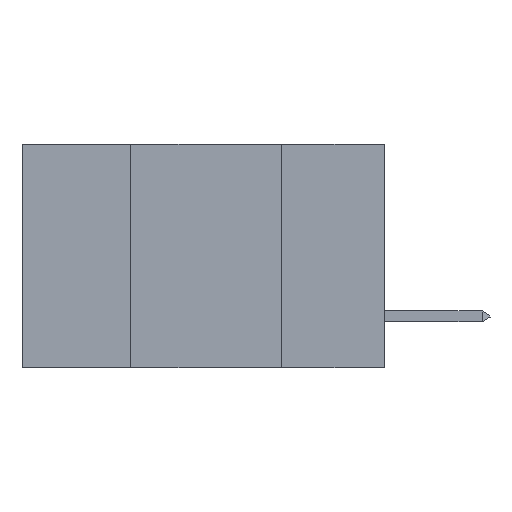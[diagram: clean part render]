
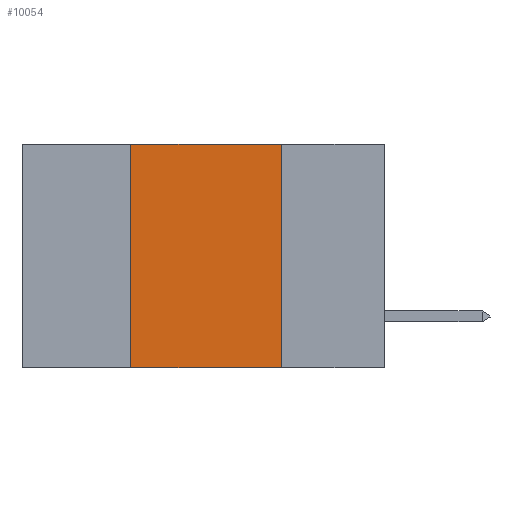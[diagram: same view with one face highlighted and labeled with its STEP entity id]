
A CAD part, left-side view. The second image highlights one B-rep face of the part: STEP entity #10054.
In plain terms, the highlighted planar face has unit normal (-1, 0, 0).
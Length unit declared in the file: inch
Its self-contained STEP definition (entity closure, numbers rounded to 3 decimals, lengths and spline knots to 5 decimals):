
#378 = DIRECTION ( 'NONE',  ( 0., -1., 0. ) ) ;
#806 = CARTESIAN_POINT ( 'NONE',  ( 0., 0.42, 0. ) ) ;
#2323 = VERTEX_POINT ( 'NONE', #33278 ) ;
#4461 = LINE ( 'NONE', #30624, #15511 ) ;
#5140 = ORIENTED_EDGE ( 'NONE', *, *, #17303, .F. ) ;
#5149 = FACE_OUTER_BOUND ( 'NONE', #28127, .T. ) ;
#9442 = VERTEX_POINT ( 'NONE', #27730 ) ;
#10054 = ADVANCED_FACE ( 'NONE', ( #5149 ), #39531, .F. ) ;
#13323 = VECTOR ( 'NONE', #378, 39.37008 ) ;
#13981 = DIRECTION ( 'NONE',  ( 0., 0., -1. ) ) ;
#13982 = CARTESIAN_POINT ( 'NONE',  ( 0., 0.6, 0. ) ) ;
#14149 = VERTEX_POINT ( 'NONE', #40591 ) ;
#14695 = DIRECTION ( 'NONE',  ( 0., 0., -1. ) ) ;
#15511 = VECTOR ( 'NONE', #14695, 39.37008 ) ;
#17303 = EDGE_CURVE ( 'NONE', #19461, #14149, #31144, .T. ) ;
#18844 = LINE ( 'NONE', #29818, #13323 ) ;
#19461 = VERTEX_POINT ( 'NONE', #806 ) ;
#20299 = CARTESIAN_POINT ( 'NONE',  ( 0., 0.6, 0. ) ) ;
#21061 = ORIENTED_EDGE ( 'NONE', *, *, #22673, .F. ) ;
#22673 = EDGE_CURVE ( 'NONE', #14149, #2323, #4461, .T. ) ;
#25546 = VECTOR ( 'NONE', #38786, 39.37008 ) ;
#26642 = DIRECTION ( 'NONE',  ( 1., 0., 0. ) ) ;
#27073 = VECTOR ( 'NONE', #37180, 39.37008 ) ;
#27730 = CARTESIAN_POINT ( 'NONE',  ( 0., 0.42, -0.37 ) ) ;
#28127 = EDGE_LOOP ( 'NONE', ( #21061, #5140, #34513, #34226 ) ) ;
#29818 = CARTESIAN_POINT ( 'NONE',  ( 0., 0.6, -0.37 ) ) ;
#30624 = CARTESIAN_POINT ( 'NONE',  ( 0., 0.17, 0. ) ) ;
#31144 = LINE ( 'NONE', #13982, #27073 ) ;
#32527 = CARTESIAN_POINT ( 'NONE',  ( 0., 0.42, 0. ) ) ;
#32604 = LINE ( 'NONE', #32527, #25546 ) ;
#33278 = CARTESIAN_POINT ( 'NONE',  ( 0., 0.17, -0.37 ) ) ;
#34226 = ORIENTED_EDGE ( 'NONE', *, *, #35246, .T. ) ;
#34513 = ORIENTED_EDGE ( 'NONE', *, *, #41514, .F. ) ;
#35246 = EDGE_CURVE ( 'NONE', #9442, #2323, #18844, .T. ) ;
#37046 = AXIS2_PLACEMENT_3D ( 'NONE', #20299, #26642, #13981 ) ;
#37180 = DIRECTION ( 'NONE',  ( 0., -1., 0. ) ) ;
#38786 = DIRECTION ( 'NONE',  ( 0., 0., 1. ) ) ;
#39531 = PLANE ( 'NONE',  #37046 ) ;
#40591 = CARTESIAN_POINT ( 'NONE',  ( 0., 0.17, 0. ) ) ;
#41514 = EDGE_CURVE ( 'NONE', #9442, #19461, #32604, .T. ) ;
